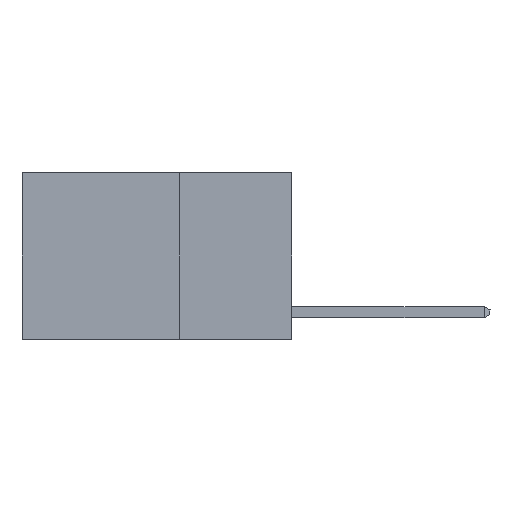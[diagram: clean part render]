
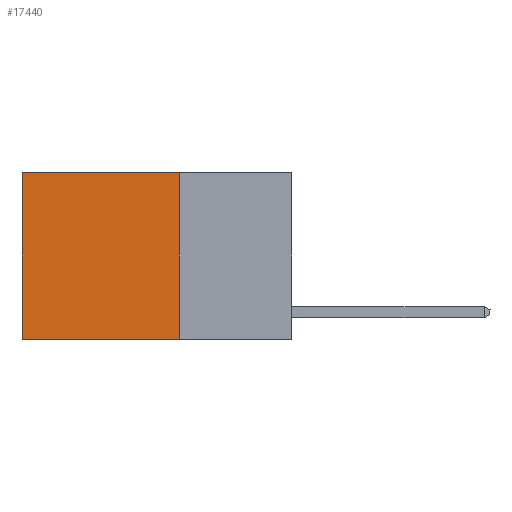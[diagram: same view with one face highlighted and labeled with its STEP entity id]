
A CAD part, left-side view. The second image highlights one B-rep face of the part: STEP entity #17440.
In plain terms, the highlighted planar face has unit normal (-1, 0, 0).
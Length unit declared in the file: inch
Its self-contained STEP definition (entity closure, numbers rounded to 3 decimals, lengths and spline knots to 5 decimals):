
#510 = EDGE_LOOP ( 'NONE', ( #2009, #527, #5571, #15797 ) ) ;
#527 = ORIENTED_EDGE ( 'NONE', *, *, #2488, .F. ) ;
#1309 = PLANE ( 'NONE',  #2805 ) ;
#1596 = VECTOR ( 'NONE', #10167, 39.37008 ) ;
#2009 = ORIENTED_EDGE ( 'NONE', *, *, #12334, .T. ) ;
#2488 = EDGE_CURVE ( 'NONE', #11216, #8474, #16530, .T. ) ;
#2805 = AXIS2_PLACEMENT_3D ( 'NONE', #5655, #14324, #5713 ) ;
#3481 = CARTESIAN_POINT ( 'NONE',  ( 0.2625, 0.6, 0. ) ) ;
#4164 = FACE_OUTER_BOUND ( 'NONE', #510, .T. ) ;
#4225 = CARTESIAN_POINT ( 'NONE',  ( 0.2625, 0.25, 0. ) ) ;
#4284 = VERTEX_POINT ( 'NONE', #16740 ) ;
#5028 = VECTOR ( 'NONE', #17420, 39.37008 ) ;
#5571 = ORIENTED_EDGE ( 'NONE', *, *, #9172, .F. ) ;
#5655 = CARTESIAN_POINT ( 'NONE',  ( 0.2625, 0.25, 0. ) ) ;
#5713 = DIRECTION ( 'NONE',  ( 0., 0., -1. ) ) ;
#5857 = CARTESIAN_POINT ( 'NONE',  ( 0.2625, 0.25, 0. ) ) ;
#5883 = CARTESIAN_POINT ( 'NONE',  ( 0.2625, 0.25, -0.37 ) ) ;
#6848 = VERTEX_POINT ( 'NONE', #4225 ) ;
#6853 = VECTOR ( 'NONE', #10616, 39.37008 ) ;
#7296 = LINE ( 'NONE', #3481, #6853 ) ;
#7388 = LINE ( 'NONE', #10666, #10769 ) ;
#8474 = VERTEX_POINT ( 'NONE', #10622 ) ;
#9172 = EDGE_CURVE ( 'NONE', #6848, #11216, #7388, .T. ) ;
#10167 = DIRECTION ( 'NONE',  ( 0., 1., 0. ) ) ;
#10616 = DIRECTION ( 'NONE',  ( 0., 0., -1. ) ) ;
#10622 = CARTESIAN_POINT ( 'NONE',  ( 0.2625, 0.6, -0.37 ) ) ;
#10666 = CARTESIAN_POINT ( 'NONE',  ( 0.2625, 0.25, 0. ) ) ;
#10769 = VECTOR ( 'NONE', #12110, 39.37008 ) ;
#11216 = VERTEX_POINT ( 'NONE', #12358 ) ;
#12110 = DIRECTION ( 'NONE',  ( 0., 0., -1. ) ) ;
#12334 = EDGE_CURVE ( 'NONE', #4284, #8474, #7296, .T. ) ;
#12358 = CARTESIAN_POINT ( 'NONE',  ( 0.2625, 0.25, -0.37 ) ) ;
#13450 = EDGE_CURVE ( 'NONE', #6848, #4284, #16539, .T. ) ;
#14324 = DIRECTION ( 'NONE',  ( 1., 0., 0. ) ) ;
#15797 = ORIENTED_EDGE ( 'NONE', *, *, #13450, .T. ) ;
#16530 = LINE ( 'NONE', #5883, #5028 ) ;
#16539 = LINE ( 'NONE', #5857, #1596 ) ;
#16740 = CARTESIAN_POINT ( 'NONE',  ( 0.2625, 0.6, 0. ) ) ;
#17420 = DIRECTION ( 'NONE',  ( 0., 1., 0. ) ) ;
#17440 = ADVANCED_FACE ( 'NONE', ( #4164 ), #1309, .F. ) ;
